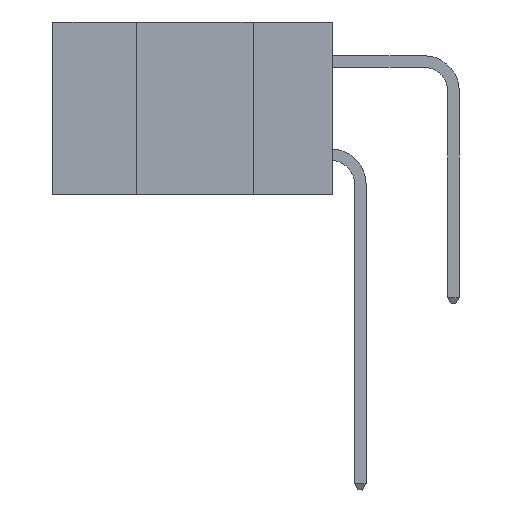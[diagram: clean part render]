
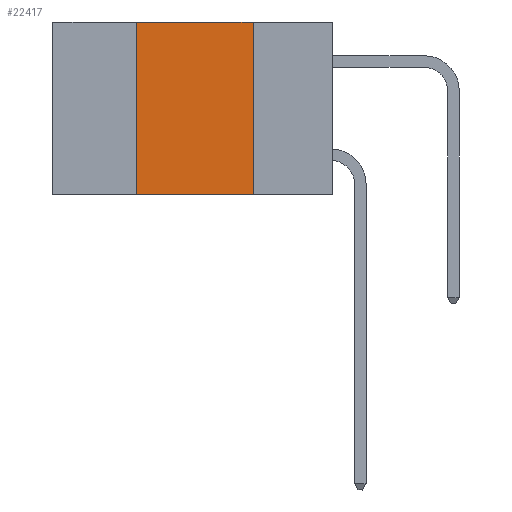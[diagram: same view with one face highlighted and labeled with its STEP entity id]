
A CAD part, left-side view. The second image highlights one B-rep face of the part: STEP entity #22417.
In plain terms, the highlighted planar face has unit normal (-1, 0, 0).
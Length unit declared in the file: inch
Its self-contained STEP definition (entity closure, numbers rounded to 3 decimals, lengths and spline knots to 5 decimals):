
#633 = EDGE_CURVE ( 'NONE', #16320, #16076, #18318, .T. ) ;
#1285 = LINE ( 'NONE', #8943, #25599 ) ;
#1383 = LINE ( 'NONE', #14844, #13866 ) ;
#1491 = CARTESIAN_POINT ( 'NONE',  ( 0., 0.6, -0.37 ) ) ;
#2309 = CARTESIAN_POINT ( 'NONE',  ( 0., 0.17, 0. ) ) ;
#3871 = PLANE ( 'NONE',  #25873 ) ;
#6159 = VECTOR ( 'NONE', #7118, 39.37008 ) ;
#6416 = CARTESIAN_POINT ( 'NONE',  ( 0., 0.42, 0. ) ) ;
#7118 = DIRECTION ( 'NONE',  ( 0., -1., 0. ) ) ;
#7453 = EDGE_LOOP ( 'NONE', ( #19805, #26464, #18839, #23198 ) ) ;
#8448 = DIRECTION ( 'NONE',  ( 1., 0., 0. ) ) ;
#8943 = CARTESIAN_POINT ( 'NONE',  ( 0., 0.17, 0. ) ) ;
#10397 = CARTESIAN_POINT ( 'NONE',  ( 0., 0.42, -0.37 ) ) ;
#11289 = DIRECTION ( 'NONE',  ( 0., -1., 0. ) ) ;
#11430 = VERTEX_POINT ( 'NONE', #10397 ) ;
#11739 = CARTESIAN_POINT ( 'NONE',  ( 0., 0.6, 0. ) ) ;
#12058 = CARTESIAN_POINT ( 'NONE',  ( 0., 0.17, -0.37 ) ) ;
#13074 = CARTESIAN_POINT ( 'NONE',  ( 0., 0.6, 0. ) ) ;
#13866 = VECTOR ( 'NONE', #24047, 39.37008 ) ;
#14844 = CARTESIAN_POINT ( 'NONE',  ( 0., 0.42, 0. ) ) ;
#15802 = EDGE_CURVE ( 'NONE', #16076, #26147, #1285, .T. ) ;
#16076 = VERTEX_POINT ( 'NONE', #2309 ) ;
#16320 = VERTEX_POINT ( 'NONE', #6416 ) ;
#17090 = DIRECTION ( 'NONE',  ( 0., 0., -1. ) ) ;
#18318 = LINE ( 'NONE', #11739, #6159 ) ;
#18839 = ORIENTED_EDGE ( 'NONE', *, *, #24428, .F. ) ;
#19805 = ORIENTED_EDGE ( 'NONE', *, *, #15802, .F. ) ;
#20349 = DIRECTION ( 'NONE',  ( 0., 0., -1. ) ) ;
#21487 = LINE ( 'NONE', #1491, #22866 ) ;
#22417 = ADVANCED_FACE ( 'NONE', ( #22703 ), #3871, .F. ) ;
#22703 = FACE_OUTER_BOUND ( 'NONE', #7453, .T. ) ;
#22866 = VECTOR ( 'NONE', #11289, 39.37008 ) ;
#23198 = ORIENTED_EDGE ( 'NONE', *, *, #25214, .T. ) ;
#24047 = DIRECTION ( 'NONE',  ( 0., 0., 1. ) ) ;
#24428 = EDGE_CURVE ( 'NONE', #11430, #16320, #1383, .T. ) ;
#25214 = EDGE_CURVE ( 'NONE', #11430, #26147, #21487, .T. ) ;
#25599 = VECTOR ( 'NONE', #20349, 39.37008 ) ;
#25873 = AXIS2_PLACEMENT_3D ( 'NONE', #13074, #8448, #17090 ) ;
#26147 = VERTEX_POINT ( 'NONE', #12058 ) ;
#26464 = ORIENTED_EDGE ( 'NONE', *, *, #633, .F. ) ;
